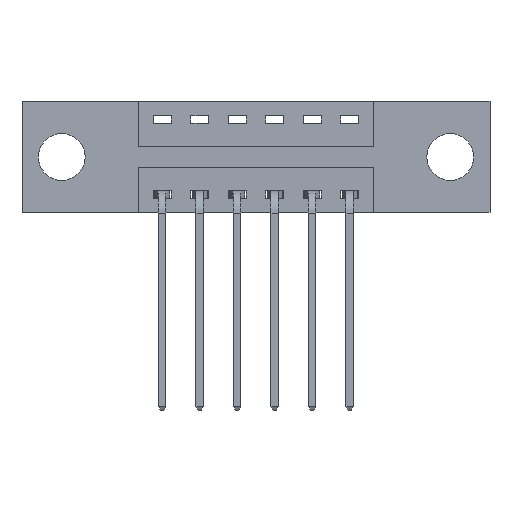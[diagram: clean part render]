
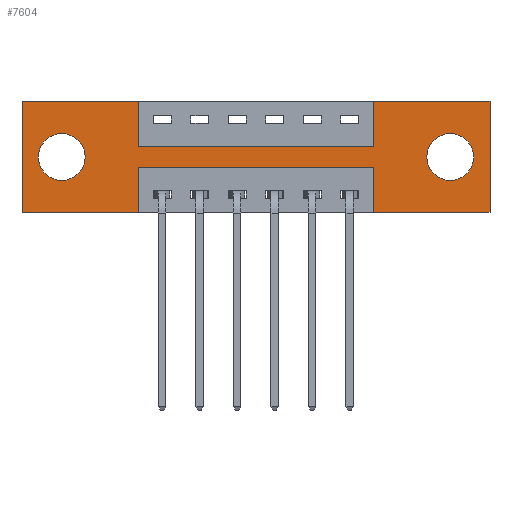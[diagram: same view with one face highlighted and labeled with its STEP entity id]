
A CAD part, front view. The second image highlights one B-rep face of the part: STEP entity #7604.
In plain terms, the highlighted planar face has unit normal (0, -1, 0).
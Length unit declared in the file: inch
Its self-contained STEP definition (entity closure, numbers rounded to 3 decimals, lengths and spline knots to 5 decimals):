
#11 = ORIENTED_EDGE ( 'NONE', *, *, #6226, .F. ) ;
#54 = ORIENTED_EDGE ( 'NONE', *, *, #4369, .F. ) ;
#242 = LINE ( 'NONE', #5805, #5348 ) ;
#246 = CARTESIAN_POINT ( 'NONE',  ( 0.3875, 0., -0.37 ) ) ;
#263 = ORIENTED_EDGE ( 'NONE', *, *, #2461, .F. ) ;
#393 = CARTESIAN_POINT ( 'NONE',  ( 0., 0., 0. ) ) ;
#451 = DIRECTION ( 'NONE',  ( 0., 0., -1. ) ) ;
#555 = VERTEX_POINT ( 'NONE', #8350 ) ;
#584 = DIRECTION ( 'NONE',  ( -1., 0., 0. ) ) ;
#713 = VERTEX_POINT ( 'NONE', #1160 ) ;
#754 = ORIENTED_EDGE ( 'NONE', *, *, #1034, .T. ) ;
#822 = DIRECTION ( 'NONE',  ( 0., 0., -1. ) ) ;
#845 = CARTESIAN_POINT ( 'NONE',  ( 1.56, 0., 0. ) ) ;
#909 = DIRECTION ( 'NONE',  ( 0., 1., 0. ) ) ;
#947 = LINE ( 'NONE', #3726, #1372 ) ;
#984 = VERTEX_POINT ( 'NONE', #2798 ) ;
#1034 = EDGE_CURVE ( 'NONE', #713, #8821, #7628, .T. ) ;
#1048 = AXIS2_PLACEMENT_3D ( 'NONE', #3177, #1911, #6711 ) ;
#1160 = CARTESIAN_POINT ( 'NONE',  ( 1.4275, 0., -0.107 ) ) ;
#1172 = CARTESIAN_POINT ( 'NONE',  ( 0.3875, 0., -0.15 ) ) ;
#1190 = CARTESIAN_POINT ( 'NONE',  ( 0., 0., -0.37 ) ) ;
#1202 = AXIS2_PLACEMENT_3D ( 'NONE', #4393, #909, #451 ) ;
#1275 = LINE ( 'NONE', #4044, #4301 ) ;
#1290 = VERTEX_POINT ( 'NONE', #5743 ) ;
#1298 = CARTESIAN_POINT ( 'NONE',  ( 1.56, 0., -0.37 ) ) ;
#1335 = VERTEX_POINT ( 'NONE', #1190 ) ;
#1372 = VECTOR ( 'NONE', #6504, 39.37008 ) ;
#1665 = DIRECTION ( 'NONE',  ( 1., 0., 0. ) ) ;
#1692 = DIRECTION ( 'NONE',  ( 0., 0., -1. ) ) ;
#1722 = CARTESIAN_POINT ( 'NONE',  ( 0., 0., -0.37 ) ) ;
#1770 = CARTESIAN_POINT ( 'NONE',  ( 0.3875, 0., 0. ) ) ;
#1796 = CIRCLE ( 'NONE', #1202, 0.078 ) ;
#1846 = AXIS2_PLACEMENT_3D ( 'NONE', #6404, #4988, #3541 ) ;
#1911 = DIRECTION ( 'NONE',  ( 0., 1., 0. ) ) ;
#1969 = LINE ( 'NONE', #6765, #8753 ) ;
#1989 = CARTESIAN_POINT ( 'NONE',  ( 0.3875, 0., -0.37 ) ) ;
#2053 = CARTESIAN_POINT ( 'NONE',  ( 1.56, 0., 0. ) ) ;
#2069 = EDGE_CURVE ( 'NONE', #4981, #7101, #947, .T. ) ;
#2234 = EDGE_CURVE ( 'NONE', #8821, #713, #1796, .T. ) ;
#2264 = CARTESIAN_POINT ( 'NONE',  ( 0.1325, 0., -0.185 ) ) ;
#2287 = VECTOR ( 'NONE', #1692, 39.37008 ) ;
#2331 = ORIENTED_EDGE ( 'NONE', *, *, #2069, .F. ) ;
#2341 = DIRECTION ( 'NONE',  ( 0., 0., -1. ) ) ;
#2392 = ORIENTED_EDGE ( 'NONE', *, *, #3717, .T. ) ;
#2461 = EDGE_CURVE ( 'NONE', #6856, #4981, #6440, .T. ) ;
#2486 = LINE ( 'NONE', #5094, #7529 ) ;
#2787 = CARTESIAN_POINT ( 'NONE',  ( 0.1325, 0., -0.263 ) ) ;
#2798 = CARTESIAN_POINT ( 'NONE',  ( 0.3875, 0., -0.15 ) ) ;
#2866 = VECTOR ( 'NONE', #7421, 39.37008 ) ;
#2895 = ORIENTED_EDGE ( 'NONE', *, *, #7987, .F. ) ;
#2929 = ORIENTED_EDGE ( 'NONE', *, *, #8751, .F. ) ;
#3124 = FACE_OUTER_BOUND ( 'NONE', #4302, .T. ) ;
#3177 = CARTESIAN_POINT ( 'NONE',  ( 1.4275, 0., -0.185 ) ) ;
#3261 = CARTESIAN_POINT ( 'NONE',  ( 1.4275, 0., -0.263 ) ) ;
#3361 = LINE ( 'NONE', #1172, #5917 ) ;
#3427 = EDGE_CURVE ( 'NONE', #7936, #1335, #5934, .T. ) ;
#3541 = DIRECTION ( 'NONE',  ( 0., 0., 1. ) ) ;
#3717 = EDGE_CURVE ( 'NONE', #6395, #1290, #4290, .T. ) ;
#3726 = CARTESIAN_POINT ( 'NONE',  ( 0., 0., -0.37 ) ) ;
#4022 = DIRECTION ( 'NONE',  ( 1., 0., 0. ) ) ;
#4044 = CARTESIAN_POINT ( 'NONE',  ( 0.3875, 0., -0.22 ) ) ;
#4048 = ORIENTED_EDGE ( 'NONE', *, *, #8110, .F. ) ;
#4143 = VERTEX_POINT ( 'NONE', #8557 ) ;
#4144 = EDGE_CURVE ( 'NONE', #1290, #6395, #5157, .T. ) ;
#4201 = VECTOR ( 'NONE', #5720, 39.37008 ) ;
#4290 = CIRCLE ( 'NONE', #5290, 0.078 ) ;
#4301 = VECTOR ( 'NONE', #584, 39.37008 ) ;
#4302 = EDGE_LOOP ( 'NONE', ( #11, #6604, #4048, #2331, #263, #54, #5557, #7162, #7546, #2895, #2929, #7953 ) ) ;
#4369 = EDGE_CURVE ( 'NONE', #6471, #6856, #2486, .T. ) ;
#4393 = CARTESIAN_POINT ( 'NONE',  ( 1.4275, 0., -0.185 ) ) ;
#4458 = VECTOR ( 'NONE', #2341, 39.37008 ) ;
#4492 = CARTESIAN_POINT ( 'NONE',  ( 0., 0., 0. ) ) ;
#4500 = FACE_BOUND ( 'NONE', #9044, .T. ) ;
#4925 = DIRECTION ( 'NONE',  ( 0., 1., 0. ) ) ;
#4961 = DIRECTION ( 'NONE',  ( 0., 0., 1. ) ) ;
#4965 = FACE_BOUND ( 'NONE', #8491, .T. ) ;
#4981 = VERTEX_POINT ( 'NONE', #1298 ) ;
#4988 = DIRECTION ( 'NONE',  ( 0., 1., 0. ) ) ;
#5094 = CARTESIAN_POINT ( 'NONE',  ( 0., 0., 0. ) ) ;
#5157 = CIRCLE ( 'NONE', #1846, 0.078 ) ;
#5213 = LINE ( 'NONE', #5770, #8610 ) ;
#5220 = DIRECTION ( 'NONE',  ( 1., 0., 0. ) ) ;
#5290 = AXIS2_PLACEMENT_3D ( 'NONE', #2264, #4925, #4961 ) ;
#5348 = VECTOR ( 'NONE', #7945, 39.37008 ) ;
#5378 = ORIENTED_EDGE ( 'NONE', *, *, #2234, .T. ) ;
#5396 = CARTESIAN_POINT ( 'NONE',  ( 0., 0., 0. ) ) ;
#5557 = ORIENTED_EDGE ( 'NONE', *, *, #8731, .F. ) ;
#5580 = CARTESIAN_POINT ( 'NONE',  ( 0.3875, 0., -0.22 ) ) ;
#5720 = DIRECTION ( 'NONE',  ( 0., 0., 1. ) ) ;
#5743 = CARTESIAN_POINT ( 'NONE',  ( 0.1325, 0., -0.107 ) ) ;
#5744 = PLANE ( 'NONE',  #7556 ) ;
#5770 = CARTESIAN_POINT ( 'NONE',  ( 1.1725, 0., 0. ) ) ;
#5805 = CARTESIAN_POINT ( 'NONE',  ( 0.3875, 0., 0. ) ) ;
#5875 = EDGE_CURVE ( 'NONE', #4143, #8321, #1275, .T. ) ;
#5917 = VECTOR ( 'NONE', #4022, 39.37008 ) ;
#5934 = LINE ( 'NONE', #6574, #2866 ) ;
#6129 = ORIENTED_EDGE ( 'NONE', *, *, #4144, .T. ) ;
#6168 = DIRECTION ( 'NONE',  ( 0., 0., 1. ) ) ;
#6226 = EDGE_CURVE ( 'NONE', #8321, #7936, #8088, .T. ) ;
#6395 = VERTEX_POINT ( 'NONE', #2787 ) ;
#6404 = CARTESIAN_POINT ( 'NONE',  ( 0.1325, 0., -0.185 ) ) ;
#6440 = LINE ( 'NONE', #845, #4458 ) ;
#6467 = DIRECTION ( 'NONE',  ( 0., -1., 0. ) ) ;
#6471 = VERTEX_POINT ( 'NONE', #8535 ) ;
#6504 = DIRECTION ( 'NONE',  ( -1., 0., 0. ) ) ;
#6574 = CARTESIAN_POINT ( 'NONE',  ( 0., 0., -0.37 ) ) ;
#6604 = ORIENTED_EDGE ( 'NONE', *, *, #5875, .F. ) ;
#6711 = DIRECTION ( 'NONE',  ( 0., 0., -1. ) ) ;
#6765 = CARTESIAN_POINT ( 'NONE',  ( 1.1725, 0., -0.37 ) ) ;
#6818 = CARTESIAN_POINT ( 'NONE',  ( 1.1725, 0., -0.37 ) ) ;
#6856 = VERTEX_POINT ( 'NONE', #2053 ) ;
#7058 = VERTEX_POINT ( 'NONE', #5396 ) ;
#7101 = VERTEX_POINT ( 'NONE', #6818 ) ;
#7110 = VECTOR ( 'NONE', #1665, 39.37008 ) ;
#7162 = ORIENTED_EDGE ( 'NONE', *, *, #7413, .F. ) ;
#7292 = LINE ( 'NONE', #393, #4201 ) ;
#7413 = EDGE_CURVE ( 'NONE', #984, #555, #3361, .T. ) ;
#7421 = DIRECTION ( 'NONE',  ( -1., 0., 0. ) ) ;
#7529 = VECTOR ( 'NONE', #5220, 39.37008 ) ;
#7546 = ORIENTED_EDGE ( 'NONE', *, *, #8505, .F. ) ;
#7556 = AXIS2_PLACEMENT_3D ( 'NONE', #1722, #6467, #822 ) ;
#7604 = ADVANCED_FACE ( 'NONE', ( #4500, #4965, #3124 ), #5744, .T. ) ;
#7628 = CIRCLE ( 'NONE', #1048, 0.078 ) ;
#7828 = LINE ( 'NONE', #4492, #7110 ) ;
#7936 = VERTEX_POINT ( 'NONE', #1989 ) ;
#7945 = DIRECTION ( 'NONE',  ( 0., 0., -1. ) ) ;
#7953 = ORIENTED_EDGE ( 'NONE', *, *, #3427, .F. ) ;
#7987 = EDGE_CURVE ( 'NONE', #7058, #8873, #7828, .T. ) ;
#8088 = LINE ( 'NONE', #246, #2287 ) ;
#8110 = EDGE_CURVE ( 'NONE', #7101, #4143, #1969, .T. ) ;
#8321 = VERTEX_POINT ( 'NONE', #5580 ) ;
#8350 = CARTESIAN_POINT ( 'NONE',  ( 1.1725, 0., -0.15 ) ) ;
#8491 = EDGE_LOOP ( 'NONE', ( #6129, #2392 ) ) ;
#8505 = EDGE_CURVE ( 'NONE', #8873, #984, #242, .T. ) ;
#8535 = CARTESIAN_POINT ( 'NONE',  ( 1.1725, 0., 0. ) ) ;
#8557 = CARTESIAN_POINT ( 'NONE',  ( 1.1725, 0., -0.22 ) ) ;
#8610 = VECTOR ( 'NONE', #8699, 39.37008 ) ;
#8699 = DIRECTION ( 'NONE',  ( 0., 0., 1. ) ) ;
#8731 = EDGE_CURVE ( 'NONE', #555, #6471, #5213, .T. ) ;
#8751 = EDGE_CURVE ( 'NONE', #1335, #7058, #7292, .T. ) ;
#8753 = VECTOR ( 'NONE', #6168, 39.37008 ) ;
#8821 = VERTEX_POINT ( 'NONE', #3261 ) ;
#8873 = VERTEX_POINT ( 'NONE', #1770 ) ;
#9044 = EDGE_LOOP ( 'NONE', ( #754, #5378 ) ) ;
